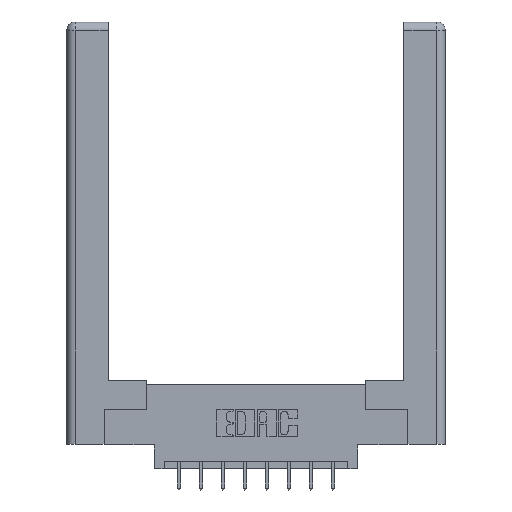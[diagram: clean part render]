
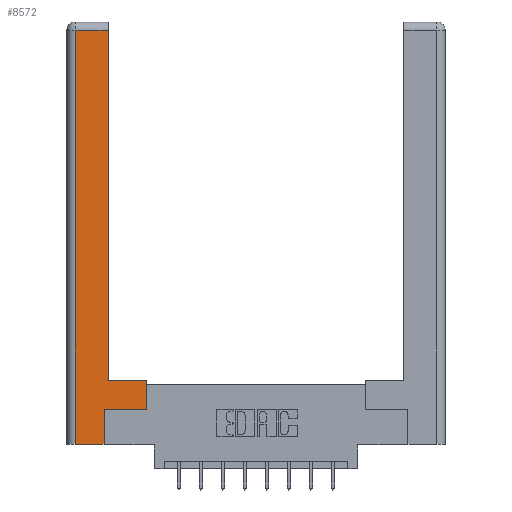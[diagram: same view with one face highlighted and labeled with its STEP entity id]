
A CAD part, top view. The second image highlights one B-rep face of the part: STEP entity #8572.
In plain terms, the highlighted planar face has unit normal (0, 0, 1).
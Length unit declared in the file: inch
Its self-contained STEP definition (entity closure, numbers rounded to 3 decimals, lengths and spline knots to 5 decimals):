
#66 = EDGE_CURVE ( 'NONE', #120, #731, #3223, .T. ) ;
#120 = VERTEX_POINT ( 'NONE', #4645 ) ;
#589 = ORIENTED_EDGE ( 'NONE', *, *, #7267, .T. ) ;
#612 = VECTOR ( 'NONE', #9109, 39.37008 ) ;
#686 = DIRECTION ( 'NONE',  ( 1., 0., 0. ) ) ;
#731 = VERTEX_POINT ( 'NONE', #4802 ) ;
#834 = LINE ( 'NONE', #5235, #4018 ) ;
#1118 = EDGE_CURVE ( 'NONE', #10483, #4416, #11348, .T. ) ;
#1130 = EDGE_LOOP ( 'NONE', ( #11364, #1867, #5337, #12892, #6198, #9015, #589, #2501 ) ) ;
#1706 = EDGE_CURVE ( 'NONE', #4069, #5814, #6290, .T. ) ;
#1867 = ORIENTED_EDGE ( 'NONE', *, *, #3693, .T. ) ;
#2132 = CARTESIAN_POINT ( 'NONE',  ( 0.0615, 0., 0. ) ) ;
#2501 = ORIENTED_EDGE ( 'NONE', *, *, #10949, .T. ) ;
#2629 = CARTESIAN_POINT ( 'NONE',  ( 0.265, 0.245, 0. ) ) ;
#2960 = CARTESIAN_POINT ( 'NONE',  ( 0.295, 0.45, 0. ) ) ;
#3223 = LINE ( 'NONE', #10720, #13173 ) ;
#3535 = VECTOR ( 'NONE', #11303, 39.37008 ) ;
#3639 = LINE ( 'NONE', #7613, #612 ) ;
#3693 = EDGE_CURVE ( 'NONE', #5814, #10483, #3639, .T. ) ;
#3710 = DIRECTION ( 'NONE',  ( 0., 0., -1. ) ) ;
#3954 = CARTESIAN_POINT ( 'NONE',  ( 0.295, 0.45, 0. ) ) ;
#4018 = VECTOR ( 'NONE', #11519, 39.37008 ) ;
#4069 = VERTEX_POINT ( 'NONE', #2960 ) ;
#4182 = EDGE_CURVE ( 'NONE', #4416, #12742, #4260, .T. ) ;
#4260 = LINE ( 'NONE', #9978, #5090 ) ;
#4416 = VERTEX_POINT ( 'NONE', #2132 ) ;
#4507 = VERTEX_POINT ( 'NONE', #10773 ) ;
#4556 = VECTOR ( 'NONE', #7824, 39.37008 ) ;
#4645 = CARTESIAN_POINT ( 'NONE',  ( 0.265, 0.245, 0. ) ) ;
#4750 = DIRECTION ( 'NONE',  ( 0., -1., 0. ) ) ;
#4802 = CARTESIAN_POINT ( 'NONE',  ( 0.565, 0.245, 0. ) ) ;
#5059 = CARTESIAN_POINT ( 'NONE',  ( 0.295, 2.94, 0. ) ) ;
#5090 = VECTOR ( 'NONE', #686, 39.37008 ) ;
#5235 = CARTESIAN_POINT ( 'NONE',  ( 0.565, 0.45, 0. ) ) ;
#5337 = ORIENTED_EDGE ( 'NONE', *, *, #1118, .T. ) ;
#5383 = FACE_OUTER_BOUND ( 'NONE', #1130, .T. ) ;
#5386 = EDGE_CURVE ( 'NONE', #12742, #120, #7514, .T. ) ;
#5814 = VERTEX_POINT ( 'NONE', #5059 ) ;
#6198 = ORIENTED_EDGE ( 'NONE', *, *, #5386, .T. ) ;
#6290 = LINE ( 'NONE', #11439, #9380 ) ;
#6300 = LINE ( 'NONE', #3954, #3535 ) ;
#6918 = DIRECTION ( 'NONE',  ( -1., 0., 0. ) ) ;
#6950 = PLANE ( 'NONE',  #10601 ) ;
#7267 = EDGE_CURVE ( 'NONE', #731, #4507, #834, .T. ) ;
#7353 = DIRECTION ( 'NONE',  ( 0., 1., 0. ) ) ;
#7405 = DIRECTION ( 'NONE',  ( 1., 0., 0. ) ) ;
#7514 = LINE ( 'NONE', #2629, #4556 ) ;
#7613 = CARTESIAN_POINT ( 'NONE',  ( 0.0615, 2.94, 0. ) ) ;
#7824 = DIRECTION ( 'NONE',  ( 0., 1., 0. ) ) ;
#8572 = ADVANCED_FACE ( 'NONE', ( #5383 ), #6950, .F. ) ;
#9015 = ORIENTED_EDGE ( 'NONE', *, *, #66, .T. ) ;
#9109 = DIRECTION ( 'NONE',  ( -1., 0., 0. ) ) ;
#9380 = VECTOR ( 'NONE', #7353, 39.37008 ) ;
#9978 = CARTESIAN_POINT ( 'NONE',  ( 0.265, 0., 0. ) ) ;
#10483 = VERTEX_POINT ( 'NONE', #11361 ) ;
#10601 = AXIS2_PLACEMENT_3D ( 'NONE', #12084, #3710, #6918 ) ;
#10635 = CARTESIAN_POINT ( 'NONE',  ( 0.265, 0., 0. ) ) ;
#10720 = CARTESIAN_POINT ( 'NONE',  ( 0.565, 0.245, 0. ) ) ;
#10773 = CARTESIAN_POINT ( 'NONE',  ( 0.565, 0.45, 0. ) ) ;
#10949 = EDGE_CURVE ( 'NONE', #4507, #4069, #6300, .T. ) ;
#11303 = DIRECTION ( 'NONE',  ( -1., 0., 0. ) ) ;
#11348 = LINE ( 'NONE', #13104, #11679 ) ;
#11361 = CARTESIAN_POINT ( 'NONE',  ( 0.0615, 2.94, 0. ) ) ;
#11364 = ORIENTED_EDGE ( 'NONE', *, *, #1706, .T. ) ;
#11439 = CARTESIAN_POINT ( 'NONE',  ( 0.295, 3., 0. ) ) ;
#11519 = DIRECTION ( 'NONE',  ( 0., 1., 0. ) ) ;
#11679 = VECTOR ( 'NONE', #4750, 39.37008 ) ;
#12084 = CARTESIAN_POINT ( 'NONE',  ( 0., 0., 0. ) ) ;
#12742 = VERTEX_POINT ( 'NONE', #10635 ) ;
#12892 = ORIENTED_EDGE ( 'NONE', *, *, #4182, .T. ) ;
#13104 = CARTESIAN_POINT ( 'NONE',  ( 0.0615, 0., 0. ) ) ;
#13173 = VECTOR ( 'NONE', #7405, 39.37008 ) ;
